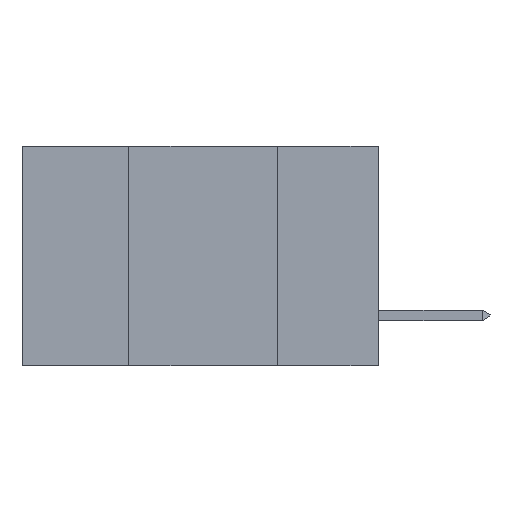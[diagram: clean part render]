
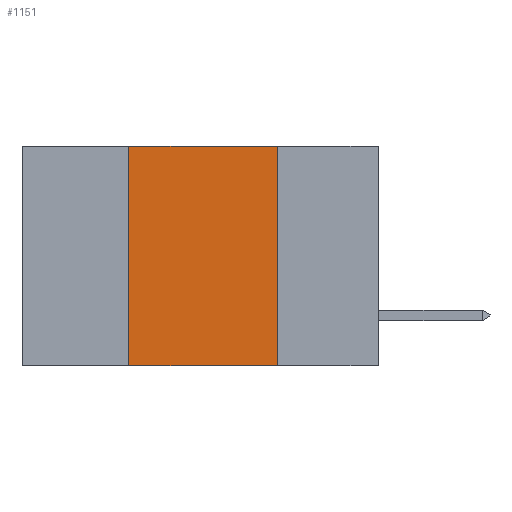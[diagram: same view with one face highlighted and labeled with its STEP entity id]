
A CAD part, left-side view. The second image highlights one B-rep face of the part: STEP entity #1151.
In plain terms, the highlighted planar face has unit normal (-1, 0, 0).
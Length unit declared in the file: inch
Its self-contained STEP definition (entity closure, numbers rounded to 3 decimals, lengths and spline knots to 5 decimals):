
#25 = EDGE_CURVE ( 'NONE', #6017, #12939, #3356, .T. ) ;
#188 = CARTESIAN_POINT ( 'NONE',  ( 0., 0.17, -0.37 ) ) ;
#371 = ORIENTED_EDGE ( 'NONE', *, *, #2788, .T. ) ;
#558 = EDGE_CURVE ( 'NONE', #12939, #3203, #5609, .T. ) ;
#1151 = ADVANCED_FACE ( 'NONE', ( #3041 ), #4540, .F. ) ;
#1317 = EDGE_CURVE ( 'NONE', #9321, #6017, #2987, .T. ) ;
#2021 = CARTESIAN_POINT ( 'NONE',  ( 0., 0.42, 0. ) ) ;
#2470 = VECTOR ( 'NONE', #6054, 39.37008 ) ;
#2771 = LINE ( 'NONE', #6695, #10921 ) ;
#2788 = EDGE_CURVE ( 'NONE', #9321, #3203, #2771, .T. ) ;
#2987 = LINE ( 'NONE', #11627, #2470 ) ;
#3041 = FACE_OUTER_BOUND ( 'NONE', #14323, .T. ) ;
#3203 = VERTEX_POINT ( 'NONE', #4403 ) ;
#3356 = LINE ( 'NONE', #13162, #8227 ) ;
#3668 = DIRECTION ( 'NONE',  ( 0., 0., -1. ) ) ;
#4403 = CARTESIAN_POINT ( 'NONE',  ( 0., 0.17, -0.37 ) ) ;
#4540 = PLANE ( 'NONE',  #9658 ) ;
#5188 = ORIENTED_EDGE ( 'NONE', *, *, #25, .F. ) ;
#5434 = CARTESIAN_POINT ( 'NONE',  ( 0., 0.17, 0. ) ) ;
#5609 = LINE ( 'NONE', #188, #6799 ) ;
#5682 = CARTESIAN_POINT ( 'NONE',  ( 0., 0.6, 0. ) ) ;
#5730 = ORIENTED_EDGE ( 'NONE', *, *, #558, .F. ) ;
#6017 = VERTEX_POINT ( 'NONE', #2021 ) ;
#6054 = DIRECTION ( 'NONE',  ( 0., 0., 1. ) ) ;
#6695 = CARTESIAN_POINT ( 'NONE',  ( 0., 0.6, -0.37 ) ) ;
#6799 = VECTOR ( 'NONE', #7991, 39.37008 ) ;
#7991 = DIRECTION ( 'NONE',  ( 0., 0., -1. ) ) ;
#8227 = VECTOR ( 'NONE', #14134, 39.37008 ) ;
#8648 = CARTESIAN_POINT ( 'NONE',  ( 0., 0.42, -0.37 ) ) ;
#9321 = VERTEX_POINT ( 'NONE', #8648 ) ;
#9658 = AXIS2_PLACEMENT_3D ( 'NONE', #5682, #11245, #3668 ) ;
#10921 = VECTOR ( 'NONE', #12366, 39.37008 ) ;
#11245 = DIRECTION ( 'NONE',  ( 1., 0., 0. ) ) ;
#11627 = CARTESIAN_POINT ( 'NONE',  ( 0., 0.42, -0.37 ) ) ;
#12366 = DIRECTION ( 'NONE',  ( 0., -1., 0. ) ) ;
#12424 = ORIENTED_EDGE ( 'NONE', *, *, #1317, .F. ) ;
#12939 = VERTEX_POINT ( 'NONE', #5434 ) ;
#13162 = CARTESIAN_POINT ( 'NONE',  ( 0., 0.6, 0. ) ) ;
#14134 = DIRECTION ( 'NONE',  ( 0., -1., 0. ) ) ;
#14323 = EDGE_LOOP ( 'NONE', ( #5730, #5188, #12424, #371 ) ) ;
